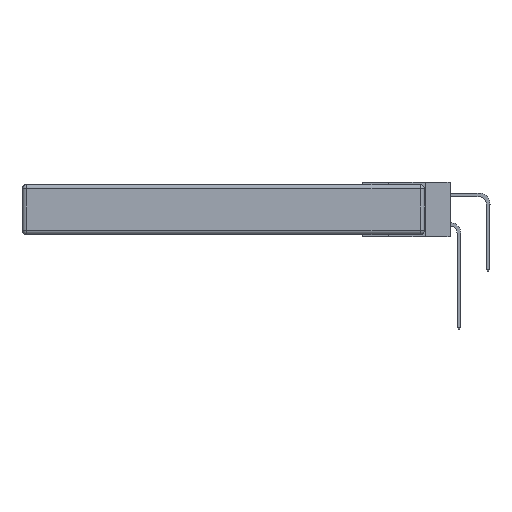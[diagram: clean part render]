
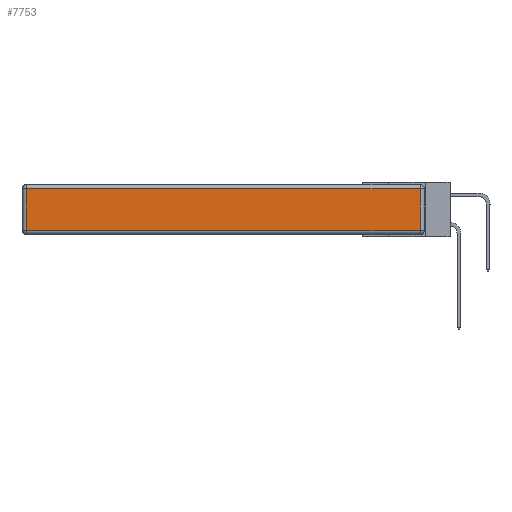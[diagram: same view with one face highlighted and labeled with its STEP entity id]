
A CAD part, left-side view. The second image highlights one B-rep face of the part: STEP entity #7753.
In plain terms, the highlighted planar face has unit normal (-1, 0, 0).
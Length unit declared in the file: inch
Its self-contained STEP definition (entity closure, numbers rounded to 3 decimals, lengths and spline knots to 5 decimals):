
#881 = DIRECTION ( 'NONE',  ( 0., 0., 1. ) ) ;
#1876 = VERTEX_POINT ( 'NONE', #24712 ) ;
#2440 = VERTEX_POINT ( 'NONE', #6561 ) ;
#2926 = DIRECTION ( 'NONE',  ( 0., 0., -1. ) ) ;
#3041 = CARTESIAN_POINT ( 'NONE',  ( 0., 0.03, -0.343 ) ) ;
#3060 = ORIENTED_EDGE ( 'NONE', *, *, #23099, .T. ) ;
#3314 = ORIENTED_EDGE ( 'NONE', *, *, #3471, .T. ) ;
#3471 = EDGE_CURVE ( 'NONE', #19555, #1876, #14057, .T. ) ;
#3541 = VECTOR ( 'NONE', #881, 39.37008 ) ;
#3645 = DIRECTION ( 'NONE',  ( 0., -1., 0. ) ) ;
#5120 = DIRECTION ( 'NONE',  ( -1., 0., 0. ) ) ;
#6561 = CARTESIAN_POINT ( 'NONE',  ( 0., 2.72, -0.313 ) ) ;
#7314 = CARTESIAN_POINT ( 'NONE',  ( 0., 0., -0.343 ) ) ;
#7496 = LINE ( 'NONE', #13631, #15469 ) ;
#7753 = ADVANCED_FACE ( 'NONE', ( #11047 ), #15583, .T. ) ;
#9344 = CARTESIAN_POINT ( 'NONE',  ( 0., 0.03, -0.313 ) ) ;
#9871 = ORIENTED_EDGE ( 'NONE', *, *, #19962, .T. ) ;
#11047 = FACE_OUTER_BOUND ( 'NONE', #14910, .T. ) ;
#11608 = DIRECTION ( 'NONE',  ( 0., 1., 0. ) ) ;
#11989 = CARTESIAN_POINT ( 'NONE',  ( 0., 2.75, -0.03 ) ) ;
#12177 = AXIS2_PLACEMENT_3D ( 'NONE', #7314, #5120, #22128 ) ;
#12210 = VECTOR ( 'NONE', #3645, 39.37008 ) ;
#12350 = CARTESIAN_POINT ( 'NONE',  ( 0., 0.03, -0.03 ) ) ;
#12534 = VERTEX_POINT ( 'NONE', #9344 ) ;
#13631 = CARTESIAN_POINT ( 'NONE',  ( 0., 2.72, -0.343 ) ) ;
#14057 = LINE ( 'NONE', #11989, #19356 ) ;
#14910 = EDGE_LOOP ( 'NONE', ( #9871, #3060, #3314, #16526 ) ) ;
#15469 = VECTOR ( 'NONE', #2926, 39.37008 ) ;
#15583 = PLANE ( 'NONE',  #12177 ) ;
#16526 = ORIENTED_EDGE ( 'NONE', *, *, #20924, .T. ) ;
#16850 = LINE ( 'NONE', #25004, #12210 ) ;
#19356 = VECTOR ( 'NONE', #11608, 39.37008 ) ;
#19555 = VERTEX_POINT ( 'NONE', #12350 ) ;
#19962 = EDGE_CURVE ( 'NONE', #2440, #12534, #16850, .T. ) ;
#20924 = EDGE_CURVE ( 'NONE', #1876, #2440, #7496, .T. ) ;
#22128 = DIRECTION ( 'NONE',  ( 0., 0., 1. ) ) ;
#23099 = EDGE_CURVE ( 'NONE', #12534, #19555, #23143, .T. ) ;
#23143 = LINE ( 'NONE', #3041, #3541 ) ;
#24712 = CARTESIAN_POINT ( 'NONE',  ( 0., 2.72, -0.03 ) ) ;
#25004 = CARTESIAN_POINT ( 'NONE',  ( 0., 0., -0.313 ) ) ;
